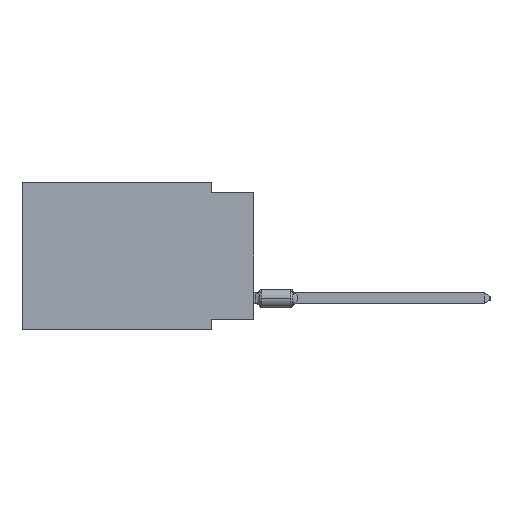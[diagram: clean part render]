
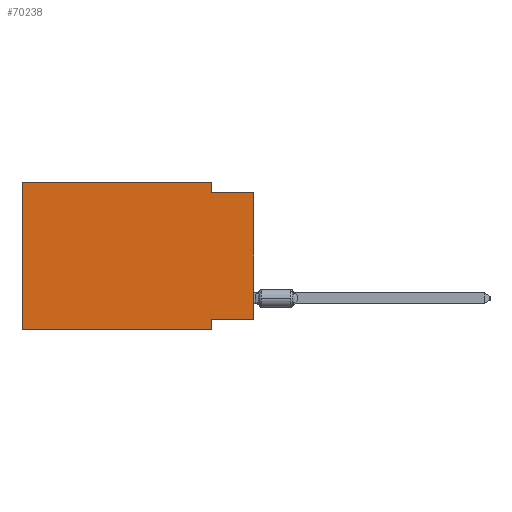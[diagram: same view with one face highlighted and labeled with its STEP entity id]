
A CAD part, left-side view. The second image highlights one B-rep face of the part: STEP entity #70238.
In plain terms, the highlighted planar face has unit normal (-1, 0, 0).
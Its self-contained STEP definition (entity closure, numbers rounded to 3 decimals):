
#227 = DIRECTION ( 'NONE',  ( 0., 0., 1. ) ) ;
#1518 = EDGE_CURVE ( 'NONE', #7937, #20715, #42615, .T. ) ;
#1793 = DIRECTION ( 'NONE',  ( 1., 0., 0. ) ) ;
#3337 = VECTOR ( 'NONE', #77822, 1000. ) ;
#3515 = CARTESIAN_POINT ( 'NONE',  ( 0., 0., -8.255 ) ) ;
#3577 = PLANE ( 'NONE',  #65973 ) ;
#6673 = CARTESIAN_POINT ( 'NONE',  ( 0., 2.54, -8.255 ) ) ;
#7832 = ORIENTED_EDGE ( 'NONE', *, *, #78832, .F. ) ;
#7937 = VERTEX_POINT ( 'NONE', #80728 ) ;
#8161 = CARTESIAN_POINT ( 'NONE',  ( 0., 2.54, 0. ) ) ;
#9933 = VECTOR ( 'NONE', #45465, 1000. ) ;
#12365 = ORIENTED_EDGE ( 'NONE', *, *, #75662, .F. ) ;
#12595 = ORIENTED_EDGE ( 'NONE', *, *, #1518, .T. ) ;
#14640 = DIRECTION ( 'NONE',  ( 0., 0., 1. ) ) ;
#15990 = DIRECTION ( 'NONE',  ( 0., 0., -1. ) ) ;
#17637 = VERTEX_POINT ( 'NONE', #56866 ) ;
#18016 = LINE ( 'NONE', #45939, #34547 ) ;
#20715 = VERTEX_POINT ( 'NONE', #31492 ) ;
#20906 = CARTESIAN_POINT ( 'NONE',  ( 0., 2.54, -0.635 ) ) ;
#23257 = LINE ( 'NONE', #8161, #49537 ) ;
#23312 = EDGE_CURVE ( 'NONE', #17637, #51620, #79776, .T. ) ;
#27334 = CARTESIAN_POINT ( 'NONE',  ( 0., 0., -0.635 ) ) ;
#28171 = CARTESIAN_POINT ( 'NONE',  ( 0., 2.54, 0. ) ) ;
#29143 = CARTESIAN_POINT ( 'NONE',  ( 0., 0., -0.635 ) ) ;
#31492 = CARTESIAN_POINT ( 'NONE',  ( 0., 2.54, -8.89 ) ) ;
#34547 = VECTOR ( 'NONE', #39080, 1000. ) ;
#35020 = CARTESIAN_POINT ( 'NONE',  ( 0., 0., 0. ) ) ;
#37006 = VERTEX_POINT ( 'NONE', #20906 ) ;
#38839 = VECTOR ( 'NONE', #227, 1000. ) ;
#39080 = DIRECTION ( 'NONE',  ( 0., 0., -1. ) ) ;
#39229 = LINE ( 'NONE', #3515, #88519 ) ;
#39710 = DIRECTION ( 'NONE',  ( 0., -1., 0. ) ) ;
#40162 = EDGE_CURVE ( 'NONE', #45559, #49471, #39229, .T. ) ;
#41615 = ORIENTED_EDGE ( 'NONE', *, *, #86829, .F. ) ;
#42615 = LINE ( 'NONE', #71414, #3337 ) ;
#43875 = DIRECTION ( 'NONE',  ( 0., 0., -1. ) ) ;
#45465 = DIRECTION ( 'NONE',  ( 0., -1., 0. ) ) ;
#45559 = VERTEX_POINT ( 'NONE', #60800 ) ;
#45939 = CARTESIAN_POINT ( 'NONE',  ( 0., 2.54, -8.89 ) ) ;
#46851 = CARTESIAN_POINT ( 'NONE',  ( 0., 13.97, 0. ) ) ;
#48756 = LINE ( 'NONE', #35020, #38839 ) ;
#49471 = VERTEX_POINT ( 'NONE', #6673 ) ;
#49537 = VECTOR ( 'NONE', #43875, 1000. ) ;
#49763 = VECTOR ( 'NONE', #39710, 1000. ) ;
#50770 = FACE_OUTER_BOUND ( 'NONE', #85643, .T. ) ;
#51620 = VERTEX_POINT ( 'NONE', #28171 ) ;
#53217 = CARTESIAN_POINT ( 'NONE',  ( 0., 13.97, 0. ) ) ;
#54949 = ORIENTED_EDGE ( 'NONE', *, *, #67520, .F. ) ;
#56866 = CARTESIAN_POINT ( 'NONE',  ( 0., 13.97, 0. ) ) ;
#58650 = ORIENTED_EDGE ( 'NONE', *, *, #86555, .T. ) ;
#59372 = DIRECTION ( 'NONE',  ( 0., 1., 0. ) ) ;
#60800 = CARTESIAN_POINT ( 'NONE',  ( 0., 0., -8.255 ) ) ;
#65282 = ORIENTED_EDGE ( 'NONE', *, *, #40162, .F. ) ;
#65973 = AXIS2_PLACEMENT_3D ( 'NONE', #78682, #1793, #15990 ) ;
#67436 = LINE ( 'NONE', #46851, #75697 ) ;
#67520 = EDGE_CURVE ( 'NONE', #37006, #81737, #68072, .T. ) ;
#68072 = LINE ( 'NONE', #27334, #49763 ) ;
#70238 = ADVANCED_FACE ( 'NONE', ( #50770 ), #3577, .F. ) ;
#71414 = CARTESIAN_POINT ( 'NONE',  ( 0., 13.97, -8.89 ) ) ;
#75662 = EDGE_CURVE ( 'NONE', #7937, #17637, #67436, .T. ) ;
#75697 = VECTOR ( 'NONE', #14640, 1000. ) ;
#76496 = ORIENTED_EDGE ( 'NONE', *, *, #23312, .F. ) ;
#77822 = DIRECTION ( 'NONE',  ( 0., -1., 0. ) ) ;
#78682 = CARTESIAN_POINT ( 'NONE',  ( 0., 13.97, 0. ) ) ;
#78832 = EDGE_CURVE ( 'NONE', #51620, #37006, #23257, .T. ) ;
#79776 = LINE ( 'NONE', #53217, #9933 ) ;
#80728 = CARTESIAN_POINT ( 'NONE',  ( 0., 13.97, -8.89 ) ) ;
#81737 = VERTEX_POINT ( 'NONE', #29143 ) ;
#85643 = EDGE_LOOP ( 'NONE', ( #58650, #54949, #7832, #76496, #12365, #12595, #41615, #65282 ) ) ;
#86555 = EDGE_CURVE ( 'NONE', #45559, #81737, #48756, .T. ) ;
#86829 = EDGE_CURVE ( 'NONE', #49471, #20715, #18016, .T. ) ;
#88519 = VECTOR ( 'NONE', #59372, 1000. ) ;
